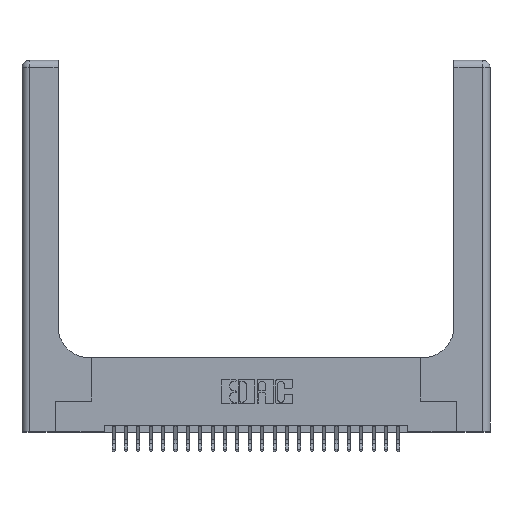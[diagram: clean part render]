
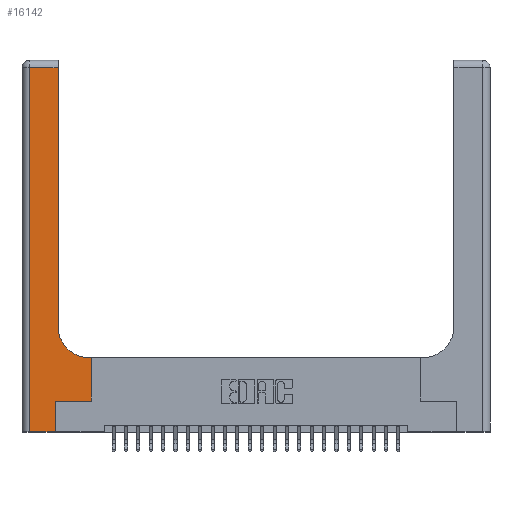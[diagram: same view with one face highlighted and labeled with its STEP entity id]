
A CAD part, top view. The second image highlights one B-rep face of the part: STEP entity #16142.
In plain terms, the highlighted planar face has unit normal (0, 0, 1).
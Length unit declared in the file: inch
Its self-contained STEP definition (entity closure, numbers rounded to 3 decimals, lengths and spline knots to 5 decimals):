
#23 = CARTESIAN_POINT ( 'NONE',  ( 0.5585, 0.25, 0.37 ) ) ;
#27 = CARTESIAN_POINT ( 'NONE',  ( 0.269, 0., 0.37 ) ) ;
#70 = VERTEX_POINT ( 'NONE', #2272 ) ;
#355 = CARTESIAN_POINT ( 'NONE',  ( 0., 0., 0.37 ) ) ;
#683 = DIRECTION ( 'NONE',  ( 1., 0., 0. ) ) ;
#921 = EDGE_CURVE ( 'NONE', #12014, #1546, #3479, .T. ) ;
#1079 = VECTOR ( 'NONE', #16333, 39.37008 ) ;
#1323 = VERTEX_POINT ( 'NONE', #26152 ) ;
#1546 = VERTEX_POINT ( 'NONE', #27 ) ;
#1855 = ORIENTED_EDGE ( 'NONE', *, *, #23981, .T. ) ;
#2093 = VECTOR ( 'NONE', #9479, 39.37008 ) ;
#2232 = DIRECTION ( 'NONE',  ( 1., 0., 0. ) ) ;
#2272 = CARTESIAN_POINT ( 'NONE',  ( 0.2915, 2.94, 0.37 ) ) ;
#2324 = FACE_OUTER_BOUND ( 'NONE', #14654, .T. ) ;
#3479 = LINE ( 'NONE', #355, #24386 ) ;
#3751 = VERTEX_POINT ( 'NONE', #7744 ) ;
#3921 = VERTEX_POINT ( 'NONE', #11789 ) ;
#4663 = VECTOR ( 'NONE', #22505, 39.37008 ) ;
#4881 = LINE ( 'NONE', #12732, #18417 ) ;
#4896 = CARTESIAN_POINT ( 'NONE',  ( 0.269, 0.25, 0.37 ) ) ;
#5124 = EDGE_CURVE ( 'NONE', #3751, #70, #4881, .T. ) ;
#5323 = LINE ( 'NONE', #5976, #1079 ) ;
#5445 = CARTESIAN_POINT ( 'NONE',  ( 0.06, 2.94, 0.37 ) ) ;
#5607 = ORIENTED_EDGE ( 'NONE', *, *, #5773, .T. ) ;
#5773 = EDGE_CURVE ( 'NONE', #70, #6215, #26245, .T. ) ;
#5968 = ORIENTED_EDGE ( 'NONE', *, *, #15034, .T. ) ;
#5976 = CARTESIAN_POINT ( 'NONE',  ( 0.2915, 0.6, 0.37 ) ) ;
#6215 = VERTEX_POINT ( 'NONE', #5445 ) ;
#6402 = EDGE_CURVE ( 'NONE', #24925, #1323, #5323, .T. ) ;
#7069 = DIRECTION ( 'NONE',  ( 1., 0., 0. ) ) ;
#7103 = CARTESIAN_POINT ( 'NONE',  ( 0.5415, 0.85, 0.37 ) ) ;
#7744 = CARTESIAN_POINT ( 'NONE',  ( 0.2915, 0.85, 0.37 ) ) ;
#7853 = EDGE_CURVE ( 'NONE', #6215, #12014, #19713, .T. ) ;
#7980 = VECTOR ( 'NONE', #20542, 39.37008 ) ;
#8182 = CARTESIAN_POINT ( 'NONE',  ( 0.269, 0., 0.37 ) ) ;
#8187 = CARTESIAN_POINT ( 'NONE',  ( 0.5585, 0.6, 0.37 ) ) ;
#8364 = LINE ( 'NONE', #9130, #15768 ) ;
#8894 = DIRECTION ( 'NONE',  ( 0., 0., -1. ) ) ;
#9130 = CARTESIAN_POINT ( 'NONE',  ( 0.269, 0.25, 0.37 ) ) ;
#9479 = DIRECTION ( 'NONE',  ( -1., 0., 0. ) ) ;
#9538 = LINE ( 'NONE', #23, #4663 ) ;
#10227 = ORIENTED_EDGE ( 'NONE', *, *, #25861, .T. ) ;
#11112 = AXIS2_PLACEMENT_3D ( 'NONE', #21329, #25513, #21504 ) ;
#11380 = VECTOR ( 'NONE', #15363, 39.37008 ) ;
#11789 = CARTESIAN_POINT ( 'NONE',  ( 0.5585, 0.25, 0.37 ) ) ;
#12014 = VERTEX_POINT ( 'NONE', #22406 ) ;
#12732 = CARTESIAN_POINT ( 'NONE',  ( 0.2915, 3., 0.37 ) ) ;
#13429 = LINE ( 'NONE', #8182, #7980 ) ;
#13962 = CARTESIAN_POINT ( 'NONE',  ( 0., 2.94, 0.37 ) ) ;
#14495 = ORIENTED_EDGE ( 'NONE', *, *, #6402, .T. ) ;
#14654 = EDGE_LOOP ( 'NONE', ( #20868, #5607, #25319, #21830, #16797, #1855, #10227, #14495, #5968 ) ) ;
#15034 = EDGE_CURVE ( 'NONE', #1323, #3751, #23644, .T. ) ;
#15363 = DIRECTION ( 'NONE',  ( 0., -1., 0. ) ) ;
#15768 = VECTOR ( 'NONE', #7069, 39.37008 ) ;
#16142 = ADVANCED_FACE ( 'NONE', ( #2324 ), #19409, .F. ) ;
#16333 = DIRECTION ( 'NONE',  ( -1., 0., 0. ) ) ;
#16797 = ORIENTED_EDGE ( 'NONE', *, *, #18838, .T. ) ;
#18417 = VECTOR ( 'NONE', #26208, 39.37008 ) ;
#18838 = EDGE_CURVE ( 'NONE', #1546, #23242, #13429, .T. ) ;
#19409 = PLANE ( 'NONE',  #11112 ) ;
#19713 = LINE ( 'NONE', #21194, #11380 ) ;
#20385 = AXIS2_PLACEMENT_3D ( 'NONE', #7103, #8894, #683 ) ;
#20542 = DIRECTION ( 'NONE',  ( 0., 1., 0. ) ) ;
#20868 = ORIENTED_EDGE ( 'NONE', *, *, #5124, .T. ) ;
#21194 = CARTESIAN_POINT ( 'NONE',  ( 0.06, 3., 0.37 ) ) ;
#21329 = CARTESIAN_POINT ( 'NONE',  ( 0., 3., 0.37 ) ) ;
#21504 = DIRECTION ( 'NONE',  ( -1., 0., 0. ) ) ;
#21830 = ORIENTED_EDGE ( 'NONE', *, *, #921, .T. ) ;
#22406 = CARTESIAN_POINT ( 'NONE',  ( 0.06, 0., 0.37 ) ) ;
#22505 = DIRECTION ( 'NONE',  ( 0., 1., 0. ) ) ;
#23242 = VERTEX_POINT ( 'NONE', #4896 ) ;
#23644 = CIRCLE ( 'NONE', #20385, 0.25 ) ;
#23981 = EDGE_CURVE ( 'NONE', #23242, #3921, #8364, .T. ) ;
#24386 = VECTOR ( 'NONE', #2232, 39.37008 ) ;
#24925 = VERTEX_POINT ( 'NONE', #8187 ) ;
#25319 = ORIENTED_EDGE ( 'NONE', *, *, #7853, .T. ) ;
#25513 = DIRECTION ( 'NONE',  ( 0., 0., -1. ) ) ;
#25861 = EDGE_CURVE ( 'NONE', #3921, #24925, #9538, .T. ) ;
#26152 = CARTESIAN_POINT ( 'NONE',  ( 0.5415, 0.6, 0.37 ) ) ;
#26208 = DIRECTION ( 'NONE',  ( 0., 1., 0. ) ) ;
#26245 = LINE ( 'NONE', #13962, #2093 ) ;
